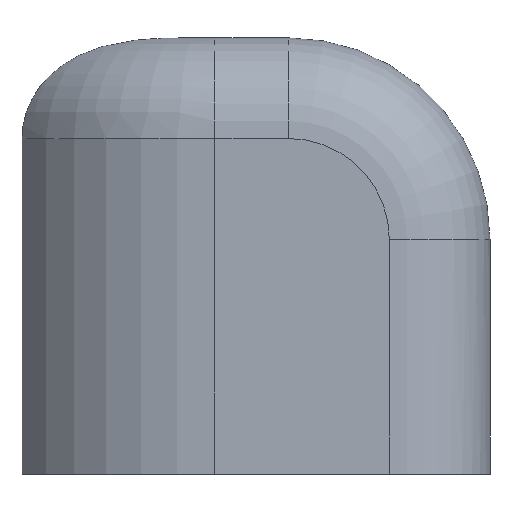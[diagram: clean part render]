
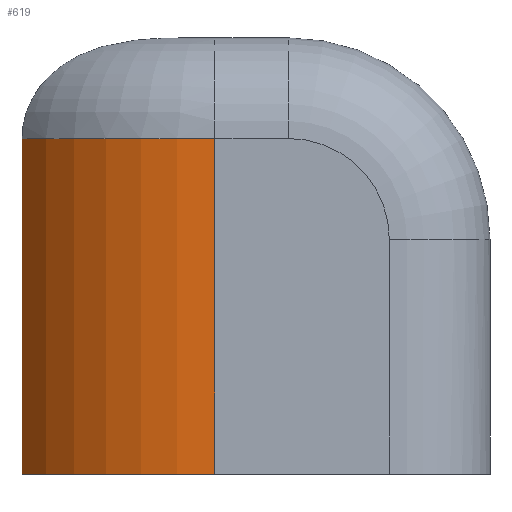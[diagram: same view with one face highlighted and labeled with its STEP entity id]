
A CAD part, left-side view. The second image highlights one B-rep face of the part: STEP entity #619.
In plain terms, the highlighted cylindrical face has radius 17.5 mm (diameter 35 mm), a partial arc.
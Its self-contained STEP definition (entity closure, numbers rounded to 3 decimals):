
#2 = CARTESIAN_POINT ( 'NONE',  ( 10., 20.5, -20. ) ) ;
#69 = VERTEX_POINT ( 'NONE', #142 ) ;
#80 = ORIENTED_EDGE ( 'NONE', *, *, #287, .F. ) ;
#127 = EDGE_CURVE ( 'NONE', #313, #501, #197, .T. ) ;
#134 = CARTESIAN_POINT ( 'NONE',  ( 10., 20.5, 5. ) ) ;
#135 = DIRECTION ( 'NONE',  ( 1., 0., 0. ) ) ;
#142 = CARTESIAN_POINT ( 'NONE',  ( 0., 34.861, 5. ) ) ;
#144 = AXIS2_PLACEMENT_3D ( 'NONE', #2, #219, #578 ) ;
#152 = CARTESIAN_POINT ( 'NONE',  ( 0., 34.861, 12.5 ) ) ;
#184 = CARTESIAN_POINT ( 'NONE',  ( 10., 20.5, 12.5 ) ) ;
#197 = LINE ( 'NONE', #596, #251 ) ;
#206 = CYLINDRICAL_SURFACE ( 'NONE', #415, 17.5 ) ;
#219 = DIRECTION ( 'NONE',  ( 0., 0., -1. ) ) ;
#224 = LINE ( 'NONE', #152, #297 ) ;
#230 = EDGE_CURVE ( 'NONE', #69, #313, #628, .T. ) ;
#251 = VECTOR ( 'NONE', #527, 1000. ) ;
#267 = FACE_OUTER_BOUND ( 'NONE', #464, .T. ) ;
#269 = ORIENTED_EDGE ( 'NONE', *, *, #127, .F. ) ;
#287 = EDGE_CURVE ( 'NONE', #501, #443, #531, .T. ) ;
#297 = VECTOR ( 'NONE', #316, 1000. ) ;
#313 = VERTEX_POINT ( 'NONE', #622 ) ;
#316 = DIRECTION ( 'NONE',  ( 0., 0., -1. ) ) ;
#364 = ORIENTED_EDGE ( 'NONE', *, *, #230, .F. ) ;
#415 = AXIS2_PLACEMENT_3D ( 'NONE', #184, #543, #502 ) ;
#443 = VERTEX_POINT ( 'NONE', #488 ) ;
#464 = EDGE_LOOP ( 'NONE', ( #586, #80, #269, #364 ) ) ;
#488 = CARTESIAN_POINT ( 'NONE',  ( 0., 34.861, -20. ) ) ;
#498 = DIRECTION ( 'NONE',  ( 0., 0., 1. ) ) ;
#501 = VERTEX_POINT ( 'NONE', #625 ) ;
#502 = DIRECTION ( 'NONE',  ( 0., 1., 0. ) ) ;
#527 = DIRECTION ( 'NONE',  ( 0., 0., -1. ) ) ;
#531 = CIRCLE ( 'NONE', #144, 17.5 ) ;
#543 = DIRECTION ( 'NONE',  ( 0., 0., -1. ) ) ;
#578 = DIRECTION ( 'NONE',  ( 0., 1., 0. ) ) ;
#586 = ORIENTED_EDGE ( 'NONE', *, *, #614, .T. ) ;
#596 = CARTESIAN_POINT ( 'NONE',  ( -7.5, 20.5, 12.5 ) ) ;
#601 = AXIS2_PLACEMENT_3D ( 'NONE', #134, #498, #135 ) ;
#614 = EDGE_CURVE ( 'NONE', #69, #443, #224, .T. ) ;
#619 = ADVANCED_FACE ( 'NONE', ( #267 ), #206, .T. ) ;
#622 = CARTESIAN_POINT ( 'NONE',  ( -7.5, 20.5, 5. ) ) ;
#625 = CARTESIAN_POINT ( 'NONE',  ( -7.5, 20.5, -20. ) ) ;
#628 = CIRCLE ( 'NONE', #601, 17.5 ) ;
